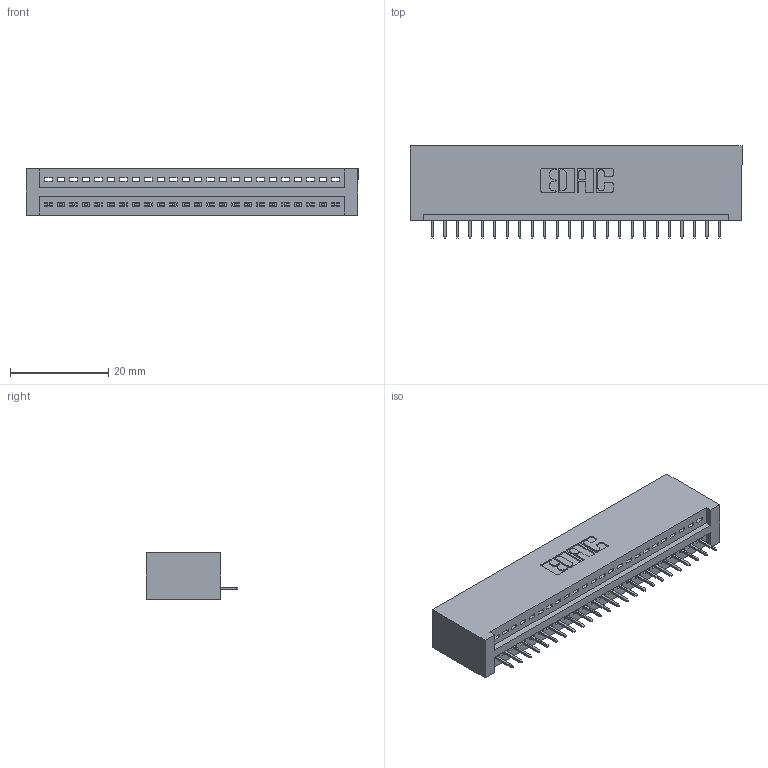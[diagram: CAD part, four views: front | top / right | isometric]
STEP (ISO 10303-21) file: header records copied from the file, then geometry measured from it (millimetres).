
FILE_DESCRIPTION (( 'STEP AP203' ), '1' );
FILE_NAME ('345-024-525-101.STEP', '2020-09-19T07:56:50', ( '' ), ( '' ), 'SwSTEP 2.0', 'SolidWorks 2020', '' );
FILE_SCHEMA (( 'CONFIG_CONTROL_DESIGN' ));
Length unit declared in the file: inch
Products named in the file (3): 345 Part_No Mounting Lugs; 345-024-525-101; 345-292-001_345-293-125
Assembly tree (25 placements, depth 2):
  345-024-525-101
    345 Part_No Mounting Lugs
    345-292-001_345-293-125  x24
Bounding box: 67.56 x 18.72 x 9.4 mm (x, y, z)
Volume: 6756.2 mm3; surface area: 8597.1 mm2
Topology: 25 solids, 25 shells, 1606 faces, 4637 edges, 2994 vertices
Faces by surface type: plane 1180, cylinder 426
Entity records: 20283 total; most frequent: CARTESIAN_POINT 3520, ORIENTED_EDGE 3478, DIRECTION 3095, EDGE_CURVE 1739, VECTOR 1523, LINE 1523, VERTEX_POINT 1154, AXIS2_PLACEMENT_3D 786
